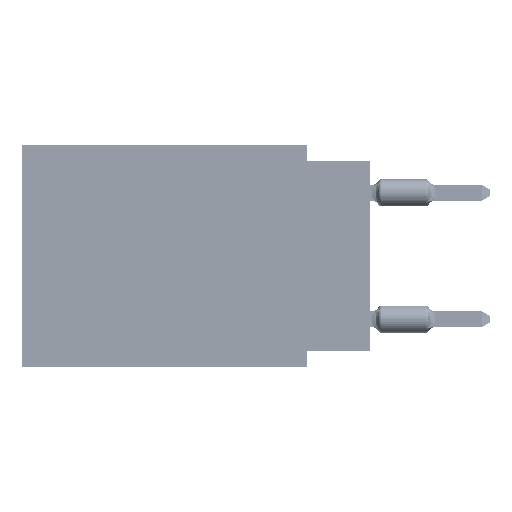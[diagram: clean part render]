
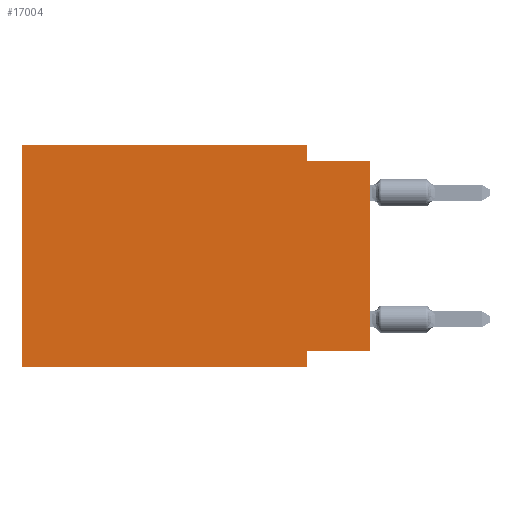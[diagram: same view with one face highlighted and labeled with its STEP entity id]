
A CAD part, left-side view. The second image highlights one B-rep face of the part: STEP entity #17004.
In plain terms, the highlighted planar face has unit normal (-1, 0, 0).
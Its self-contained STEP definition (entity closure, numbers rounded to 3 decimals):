
#429 = LINE ( 'NONE', #19324, #65142 ) ;
#447 = EDGE_CURVE ( 'NONE', #60885, #12065, #73035, .T. ) ;
#1402 = DIRECTION ( 'NONE',  ( 0., 0., -1. ) ) ;
#1579 = FACE_OUTER_BOUND ( 'NONE', #18643, .T. ) ;
#2351 = ORIENTED_EDGE ( 'NONE', *, *, #3785, .F. ) ;
#3575 = CARTESIAN_POINT ( 'NONE',  ( 0., 0., -8.255 ) ) ;
#3580 = VERTEX_POINT ( 'NONE', #30492 ) ;
#3785 = EDGE_CURVE ( 'NONE', #57705, #62873, #66916, .T. ) ;
#5105 = CARTESIAN_POINT ( 'NONE',  ( 0., 13.97, -8.89 ) ) ;
#5335 = EDGE_CURVE ( 'NONE', #62873, #3580, #429, .T. ) ;
#6267 = VECTOR ( 'NONE', #43050, 1000. ) ;
#9987 = VECTOR ( 'NONE', #1402, 1000. ) ;
#10701 = CARTESIAN_POINT ( 'NONE',  ( 0., 13.97, 0. ) ) ;
#12065 = VERTEX_POINT ( 'NONE', #61242 ) ;
#15395 = DIRECTION ( 'NONE',  ( 1., 0., 0. ) ) ;
#17004 = ADVANCED_FACE ( 'NONE', ( #1579 ), #40210, .F. ) ;
#18643 = EDGE_LOOP ( 'NONE', ( #24026, #37243, #2351, #55643, #22356, #19918, #66520, #47264 ) ) ;
#19324 = CARTESIAN_POINT ( 'NONE',  ( 0., 0., -0.635 ) ) ;
#19918 = ORIENTED_EDGE ( 'NONE', *, *, #23461, .T. ) ;
#22356 = ORIENTED_EDGE ( 'NONE', *, *, #31165, .F. ) ;
#23360 = EDGE_CURVE ( 'NONE', #50381, #60885, #41826, .T. ) ;
#23461 = EDGE_CURVE ( 'NONE', #76791, #12065, #48131, .T. ) ;
#24026 = ORIENTED_EDGE ( 'NONE', *, *, #28954, .T. ) ;
#27864 = CARTESIAN_POINT ( 'NONE',  ( 0., 2.54, -8.255 ) ) ;
#28954 = EDGE_CURVE ( 'NONE', #50381, #3580, #76384, .T. ) ;
#30451 = VECTOR ( 'NONE', #52319, 1000. ) ;
#30492 = CARTESIAN_POINT ( 'NONE',  ( 0., 0., -0.635 ) ) ;
#31165 = EDGE_CURVE ( 'NONE', #76791, #71472, #54206, .T. ) ;
#32668 = AXIS2_PLACEMENT_3D ( 'NONE', #45707, #15395, #66674 ) ;
#32751 = DIRECTION ( 'NONE',  ( 0., -1., 0. ) ) ;
#35638 = CARTESIAN_POINT ( 'NONE',  ( 0., 2.54, -0.635 ) ) ;
#37243 = ORIENTED_EDGE ( 'NONE', *, *, #5335, .F. ) ;
#37988 = DIRECTION ( 'NONE',  ( 0., -1., 0. ) ) ;
#39503 = DIRECTION ( 'NONE',  ( 0., 0., 1. ) ) ;
#40210 = PLANE ( 'NONE',  #32668 ) ;
#40271 = CARTESIAN_POINT ( 'NONE',  ( 0., 2.54, -8.89 ) ) ;
#41086 = DIRECTION ( 'NONE',  ( 0., 0., -1. ) ) ;
#41826 = LINE ( 'NONE', #3575, #48260 ) ;
#42223 = DIRECTION ( 'NONE',  ( 0., 1., 0. ) ) ;
#43050 = DIRECTION ( 'NONE',  ( 0., -1., 0. ) ) ;
#45707 = CARTESIAN_POINT ( 'NONE',  ( 0., 13.97, 0. ) ) ;
#46230 = CARTESIAN_POINT ( 'NONE',  ( 0., 13.97, 0. ) ) ;
#47264 = ORIENTED_EDGE ( 'NONE', *, *, #23360, .F. ) ;
#48131 = LINE ( 'NONE', #73757, #80448 ) ;
#48260 = VECTOR ( 'NONE', #42223, 1000. ) ;
#49774 = LINE ( 'NONE', #10701, #6267 ) ;
#49819 = VECTOR ( 'NONE', #41086, 1000. ) ;
#50008 = CARTESIAN_POINT ( 'NONE',  ( 0., 13.97, 0. ) ) ;
#50381 = VERTEX_POINT ( 'NONE', #62338 ) ;
#52319 = DIRECTION ( 'NONE',  ( 0., 0., 1. ) ) ;
#54206 = LINE ( 'NONE', #46230, #80211 ) ;
#55643 = ORIENTED_EDGE ( 'NONE', *, *, #57659, .F. ) ;
#57659 = EDGE_CURVE ( 'NONE', #71472, #57705, #49774, .T. ) ;
#57705 = VERTEX_POINT ( 'NONE', #63216 ) ;
#58970 = CARTESIAN_POINT ( 'NONE',  ( 0., 2.54, 0. ) ) ;
#60885 = VERTEX_POINT ( 'NONE', #27864 ) ;
#61242 = CARTESIAN_POINT ( 'NONE',  ( 0., 2.54, -8.89 ) ) ;
#62338 = CARTESIAN_POINT ( 'NONE',  ( 0., 0., -8.255 ) ) ;
#62873 = VERTEX_POINT ( 'NONE', #35638 ) ;
#63216 = CARTESIAN_POINT ( 'NONE',  ( 0., 2.54, 0. ) ) ;
#65142 = VECTOR ( 'NONE', #32751, 1000. ) ;
#66520 = ORIENTED_EDGE ( 'NONE', *, *, #447, .F. ) ;
#66674 = DIRECTION ( 'NONE',  ( 0., 0., -1. ) ) ;
#66916 = LINE ( 'NONE', #58970, #9987 ) ;
#70089 = CARTESIAN_POINT ( 'NONE',  ( 0., 0., 0. ) ) ;
#71472 = VERTEX_POINT ( 'NONE', #50008 ) ;
#73035 = LINE ( 'NONE', #40271, #49819 ) ;
#73757 = CARTESIAN_POINT ( 'NONE',  ( 0., 13.97, -8.89 ) ) ;
#76384 = LINE ( 'NONE', #70089, #30451 ) ;
#76791 = VERTEX_POINT ( 'NONE', #5105 ) ;
#80211 = VECTOR ( 'NONE', #39503, 1000. ) ;
#80448 = VECTOR ( 'NONE', #37988, 1000. ) ;
